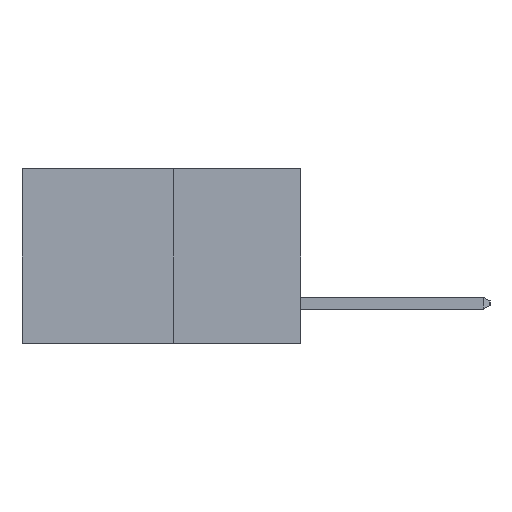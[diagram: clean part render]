
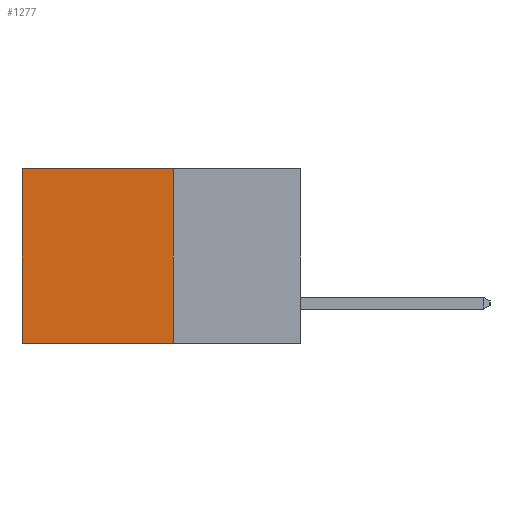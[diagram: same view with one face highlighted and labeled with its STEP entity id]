
A CAD part, left-side view. The second image highlights one B-rep face of the part: STEP entity #1277.
In plain terms, the highlighted planar face has unit normal (-1, 0, 0).
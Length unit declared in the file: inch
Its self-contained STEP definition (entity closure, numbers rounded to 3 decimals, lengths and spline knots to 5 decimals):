
#31 = VERTEX_POINT ( 'NONE', #1194 ) ;
#1194 = CARTESIAN_POINT ( 'NONE',  ( 0.277, 0.59, 0. ) ) ;
#1225 = CARTESIAN_POINT ( 'NONE',  ( 0.277, 0.27, -0.37 ) ) ;
#1277 = ADVANCED_FACE ( 'NONE', ( #8474 ), #2477, .F. ) ;
#1553 = LINE ( 'NONE', #5632, #9536 ) ;
#1582 = EDGE_LOOP ( 'NONE', ( #4040, #12514, #10016, #2301 ) ) ;
#2168 = CARTESIAN_POINT ( 'NONE',  ( 0.277, 0.27, 0. ) ) ;
#2259 = VERTEX_POINT ( 'NONE', #13339 ) ;
#2301 = ORIENTED_EDGE ( 'NONE', *, *, #10811, .T. ) ;
#2439 = DIRECTION ( 'NONE',  ( 0., 0., -1. ) ) ;
#2477 = PLANE ( 'NONE',  #4717 ) ;
#4040 = ORIENTED_EDGE ( 'NONE', *, *, #4228, .T. ) ;
#4228 = EDGE_CURVE ( 'NONE', #31, #2259, #6341, .T. ) ;
#4717 = AXIS2_PLACEMENT_3D ( 'NONE', #10620, #8026, #7993 ) ;
#4880 = CARTESIAN_POINT ( 'NONE',  ( 0.277, 0.27, -0.37 ) ) ;
#5632 = CARTESIAN_POINT ( 'NONE',  ( 0.277, 0.27, -0.37 ) ) ;
#6191 = CARTESIAN_POINT ( 'NONE',  ( 0.277, 0.59, -0.37 ) ) ;
#6236 = DIRECTION ( 'NONE',  ( 0., 0., -1. ) ) ;
#6341 = LINE ( 'NONE', #6191, #11638 ) ;
#6447 = VERTEX_POINT ( 'NONE', #4880 ) ;
#7922 = VERTEX_POINT ( 'NONE', #2168 ) ;
#7962 = CARTESIAN_POINT ( 'NONE',  ( 0.277, 0.27, 0. ) ) ;
#7993 = DIRECTION ( 'NONE',  ( 0., 0., -1. ) ) ;
#8026 = DIRECTION ( 'NONE',  ( 1., 0., 0. ) ) ;
#8064 = VECTOR ( 'NONE', #11070, 39.37008 ) ;
#8474 = FACE_OUTER_BOUND ( 'NONE', #1582, .T. ) ;
#9536 = VECTOR ( 'NONE', #13002, 39.37008 ) ;
#9565 = LINE ( 'NONE', #1225, #12027 ) ;
#9931 = EDGE_CURVE ( 'NONE', #7922, #6447, #9565, .T. ) ;
#10016 = ORIENTED_EDGE ( 'NONE', *, *, #9931, .F. ) ;
#10620 = CARTESIAN_POINT ( 'NONE',  ( 0.277, 0.27, -0.37 ) ) ;
#10811 = EDGE_CURVE ( 'NONE', #7922, #31, #10875, .T. ) ;
#10875 = LINE ( 'NONE', #7962, #8064 ) ;
#11070 = DIRECTION ( 'NONE',  ( 0., 1., 0. ) ) ;
#11638 = VECTOR ( 'NONE', #6236, 39.37008 ) ;
#12027 = VECTOR ( 'NONE', #2439, 39.37008 ) ;
#12514 = ORIENTED_EDGE ( 'NONE', *, *, #12706, .F. ) ;
#12706 = EDGE_CURVE ( 'NONE', #6447, #2259, #1553, .T. ) ;
#13002 = DIRECTION ( 'NONE',  ( 0., 1., 0. ) ) ;
#13339 = CARTESIAN_POINT ( 'NONE',  ( 0.277, 0.59, -0.37 ) ) ;
